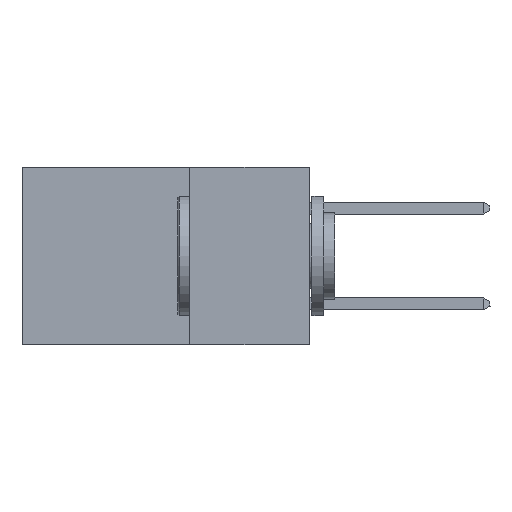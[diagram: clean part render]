
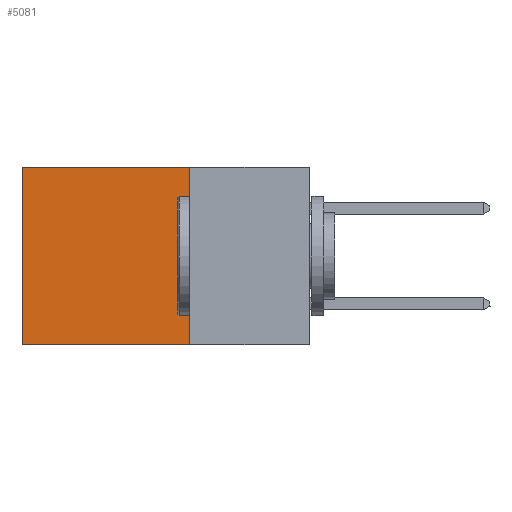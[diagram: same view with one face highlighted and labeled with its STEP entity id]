
A CAD part, left-side view. The second image highlights one B-rep face of the part: STEP entity #5081.
In plain terms, the highlighted planar face has unit normal (-1, 0, 0).
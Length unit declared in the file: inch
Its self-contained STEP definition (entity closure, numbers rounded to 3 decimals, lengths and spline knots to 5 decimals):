
#99 = CARTESIAN_POINT ( 'NONE',  ( 0.2875, 0.6, 0. ) ) ;
#1414 = VECTOR ( 'NONE', #34566, 39.37008 ) ;
#1870 = EDGE_CURVE ( 'NONE', #30848, #15475, #14599, .T. ) ;
#2524 = ORIENTED_EDGE ( 'NONE', *, *, #28710, .T. ) ;
#3506 = LINE ( 'NONE', #10599, #22020 ) ;
#3797 = EDGE_LOOP ( 'NONE', ( #2524, #20726, #22692, #32962 ) ) ;
#3997 = CARTESIAN_POINT ( 'NONE',  ( 0.2875, 0.25, 0. ) ) ;
#5081 = ADVANCED_FACE ( 'NONE', ( #20900 ), #18192, .F. ) ;
#7019 = LINE ( 'NONE', #12435, #1414 ) ;
#8015 = CARTESIAN_POINT ( 'NONE',  ( 0.2875, 0.6, -0.37 ) ) ;
#9970 = VECTOR ( 'NONE', #17745, 39.37008 ) ;
#10012 = DIRECTION ( 'NONE',  ( 1., 0., 0. ) ) ;
#10599 = CARTESIAN_POINT ( 'NONE',  ( 0.2875, 0.6, 0. ) ) ;
#12435 = CARTESIAN_POINT ( 'NONE',  ( 0.2875, 0.25, 0. ) ) ;
#12616 = CARTESIAN_POINT ( 'NONE',  ( 0.2875, 0.25, -0.37 ) ) ;
#14427 = VERTEX_POINT ( 'NONE', #3997 ) ;
#14599 = LINE ( 'NONE', #20557, #35569 ) ;
#15475 = VERTEX_POINT ( 'NONE', #8015 ) ;
#16234 = DIRECTION ( 'NONE',  ( 0., 0., -1. ) ) ;
#16294 = EDGE_CURVE ( 'NONE', #14427, #30848, #32248, .T. ) ;
#17456 = VERTEX_POINT ( 'NONE', #99 ) ;
#17670 = EDGE_CURVE ( 'NONE', #14427, #17456, #7019, .T. ) ;
#17745 = DIRECTION ( 'NONE',  ( 0., 0., -1. ) ) ;
#18192 = PLANE ( 'NONE',  #24138 ) ;
#20557 = CARTESIAN_POINT ( 'NONE',  ( 0.2875, 0.25, -0.37 ) ) ;
#20726 = ORIENTED_EDGE ( 'NONE', *, *, #1870, .F. ) ;
#20900 = FACE_OUTER_BOUND ( 'NONE', #3797, .T. ) ;
#22020 = VECTOR ( 'NONE', #16234, 39.37008 ) ;
#22692 = ORIENTED_EDGE ( 'NONE', *, *, #16294, .F. ) ;
#24138 = AXIS2_PLACEMENT_3D ( 'NONE', #26557, #10012, #29175 ) ;
#26557 = CARTESIAN_POINT ( 'NONE',  ( 0.2875, 0.25, 0. ) ) ;
#28710 = EDGE_CURVE ( 'NONE', #17456, #15475, #3506, .T. ) ;
#29175 = DIRECTION ( 'NONE',  ( 0., 0., -1. ) ) ;
#30848 = VERTEX_POINT ( 'NONE', #12616 ) ;
#31439 = DIRECTION ( 'NONE',  ( 0., 1., 0. ) ) ;
#32248 = LINE ( 'NONE', #33800, #9970 ) ;
#32962 = ORIENTED_EDGE ( 'NONE', *, *, #17670, .T. ) ;
#33800 = CARTESIAN_POINT ( 'NONE',  ( 0.2875, 0.25, 0. ) ) ;
#34566 = DIRECTION ( 'NONE',  ( 0., 1., 0. ) ) ;
#35569 = VECTOR ( 'NONE', #31439, 39.37008 ) ;
